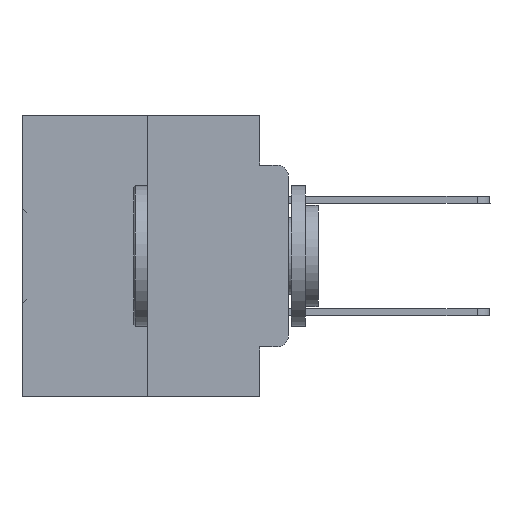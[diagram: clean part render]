
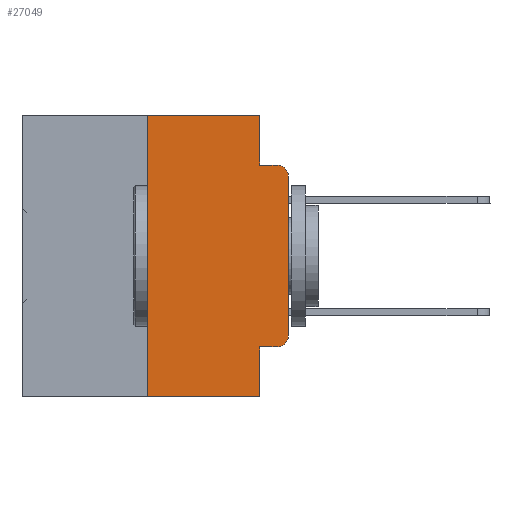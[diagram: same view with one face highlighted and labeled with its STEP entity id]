
A CAD part, left-side view. The second image highlights one B-rep face of the part: STEP entity #27049.
In plain terms, the highlighted planar face has unit normal (-1, 0, 0).
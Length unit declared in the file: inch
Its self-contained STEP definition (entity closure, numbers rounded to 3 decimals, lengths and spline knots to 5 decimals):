
#263 = CARTESIAN_POINT ( 'NONE',  ( 0., 0.051, -0.4115 ) ) ;
#491 = VERTEX_POINT ( 'NONE', #30525 ) ;
#602 = CARTESIAN_POINT ( 'NONE',  ( 0., 0.25, -0.5 ) ) ;
#1112 = DIRECTION ( 'NONE',  ( 0., 0., -1. ) ) ;
#1123 = DIRECTION ( 'NONE',  ( 0., -1., 0. ) ) ;
#1315 = ORIENTED_EDGE ( 'NONE', *, *, #19441, .T. ) ;
#2215 = CARTESIAN_POINT ( 'NONE',  ( 0., 0.02, -0.1085 ) ) ;
#2523 = DIRECTION ( 'NONE',  ( 0., 0., 1. ) ) ;
#2767 = ORIENTED_EDGE ( 'NONE', *, *, #11014, .F. ) ;
#2923 = VERTEX_POINT ( 'NONE', #30788 ) ;
#3216 = VERTEX_POINT ( 'NONE', #3576 ) ;
#3576 = CARTESIAN_POINT ( 'NONE',  ( 0., 0.02, -0.4115 ) ) ;
#4237 = EDGE_CURVE ( 'NONE', #9511, #13830, #15731, .T. ) ;
#4413 = ORIENTED_EDGE ( 'NONE', *, *, #8014, .T. ) ;
#5120 = LINE ( 'NONE', #29981, #7743 ) ;
#5161 = CARTESIAN_POINT ( 'NONE',  ( 0., 0.051, -0.4115 ) ) ;
#6084 = VERTEX_POINT ( 'NONE', #8477 ) ;
#6531 = LINE ( 'NONE', #29184, #16948 ) ;
#7331 = ORIENTED_EDGE ( 'NONE', *, *, #21489, .F. ) ;
#7436 = DIRECTION ( 'NONE',  ( 0., 0., 1. ) ) ;
#7743 = VECTOR ( 'NONE', #7436, 39.37008 ) ;
#7784 = AXIS2_PLACEMENT_3D ( 'NONE', #8228, #27696, #29920 ) ;
#8014 = EDGE_CURVE ( 'NONE', #3216, #491, #21829, .T. ) ;
#8165 = VECTOR ( 'NONE', #2523, 39.37008 ) ;
#8228 = CARTESIAN_POINT ( 'NONE',  ( 0., 0.473, 0. ) ) ;
#8248 = ORIENTED_EDGE ( 'NONE', *, *, #23022, .F. ) ;
#8477 = CARTESIAN_POINT ( 'NONE',  ( 0., 0.051, -0.0885 ) ) ;
#9511 = VERTEX_POINT ( 'NONE', #602 ) ;
#10526 = DIRECTION ( 'NONE',  ( -1., 0., 0. ) ) ;
#10883 = DIRECTION ( 'NONE',  ( 0., -1., 0. ) ) ;
#11014 = EDGE_CURVE ( 'NONE', #18075, #2923, #6531, .T. ) ;
#11150 = EDGE_CURVE ( 'NONE', #11216, #31219, #32682, .T. ) ;
#11216 = VERTEX_POINT ( 'NONE', #18666 ) ;
#11262 = EDGE_CURVE ( 'NONE', #28869, #3216, #24409, .T. ) ;
#11607 = DIRECTION ( 'NONE',  ( 0., -1., 0. ) ) ;
#11678 = LINE ( 'NONE', #14101, #14292 ) ;
#11853 = ORIENTED_EDGE ( 'NONE', *, *, #27404, .F. ) ;
#12034 = ORIENTED_EDGE ( 'NONE', *, *, #11150, .T. ) ;
#12565 = AXIS2_PLACEMENT_3D ( 'NONE', #12947, #19152, #1112 ) ;
#12947 = CARTESIAN_POINT ( 'NONE',  ( 0., 0.02, -0.3915 ) ) ;
#13374 = DIRECTION ( 'NONE',  ( 0., 0., -1. ) ) ;
#13830 = VERTEX_POINT ( 'NONE', #25325 ) ;
#14101 = CARTESIAN_POINT ( 'NONE',  ( 0., 0.051, 0. ) ) ;
#14292 = VECTOR ( 'NONE', #19574, 39.37008 ) ;
#15259 = VECTOR ( 'NONE', #10883, 39.37008 ) ;
#15731 = LINE ( 'NONE', #34508, #18341 ) ;
#16223 = PLANE ( 'NONE',  #7784 ) ;
#16948 = VECTOR ( 'NONE', #29052, 39.37008 ) ;
#18075 = VERTEX_POINT ( 'NONE', #31237 ) ;
#18341 = VECTOR ( 'NONE', #1123, 39.37008 ) ;
#18666 = CARTESIAN_POINT ( 'NONE',  ( 0., 0., -0.1085 ) ) ;
#18863 = ORIENTED_EDGE ( 'NONE', *, *, #19677, .F. ) ;
#19147 = DIRECTION ( 'NONE',  ( 0., 0., -1. ) ) ;
#19152 = DIRECTION ( 'NONE',  ( -1., 0., 0. ) ) ;
#19441 = EDGE_CURVE ( 'NONE', #491, #11216, #5120, .T. ) ;
#19447 = CARTESIAN_POINT ( 'NONE',  ( 0., 0.25, 0. ) ) ;
#19574 = DIRECTION ( 'NONE',  ( 0., 0., -1. ) ) ;
#19677 = EDGE_CURVE ( 'NONE', #9511, #18075, #32994, .T. ) ;
#21489 = EDGE_CURVE ( 'NONE', #28869, #13830, #11678, .T. ) ;
#21829 = CIRCLE ( 'NONE', #12565, 0.02 ) ;
#22908 = CARTESIAN_POINT ( 'NONE',  ( 0., 0.051, -0.0885 ) ) ;
#23022 = EDGE_CURVE ( 'NONE', #2923, #6084, #31638, .T. ) ;
#23381 = AXIS2_PLACEMENT_3D ( 'NONE', #2215, #10526, #19147 ) ;
#23522 = EDGE_LOOP ( 'NONE', ( #1315, #12034, #11853, #8248, #2767, #18863, #31347, #7331, #28934, #4413 ) ) ;
#24409 = LINE ( 'NONE', #5161, #15259 ) ;
#25325 = CARTESIAN_POINT ( 'NONE',  ( 0., 0.051, -0.5 ) ) ;
#27049 = ADVANCED_FACE ( 'NONE', ( #33118 ), #16223, .F. ) ;
#27404 = EDGE_CURVE ( 'NONE', #6084, #31219, #31792, .T. ) ;
#27427 = VECTOR ( 'NONE', #11607, 39.37008 ) ;
#27696 = DIRECTION ( 'NONE',  ( 1., 0., 0. ) ) ;
#28869 = VERTEX_POINT ( 'NONE', #263 ) ;
#28934 = ORIENTED_EDGE ( 'NONE', *, *, #11262, .T. ) ;
#29052 = DIRECTION ( 'NONE',  ( 0., -1., 0. ) ) ;
#29184 = CARTESIAN_POINT ( 'NONE',  ( 0., 0.473, 0. ) ) ;
#29920 = DIRECTION ( 'NONE',  ( 0., 0., -1. ) ) ;
#29981 = CARTESIAN_POINT ( 'NONE',  ( 0., 0., 0. ) ) ;
#30525 = CARTESIAN_POINT ( 'NONE',  ( 0., 0., -0.3915 ) ) ;
#30788 = CARTESIAN_POINT ( 'NONE',  ( 0., 0.051, 0. ) ) ;
#31219 = VERTEX_POINT ( 'NONE', #34226 ) ;
#31237 = CARTESIAN_POINT ( 'NONE',  ( 0., 0.25, 0. ) ) ;
#31347 = ORIENTED_EDGE ( 'NONE', *, *, #4237, .T. ) ;
#31638 = LINE ( 'NONE', #33112, #35553 ) ;
#31792 = LINE ( 'NONE', #22908, #27427 ) ;
#32682 = CIRCLE ( 'NONE', #23381, 0.02 ) ;
#32994 = LINE ( 'NONE', #19447, #8165 ) ;
#33112 = CARTESIAN_POINT ( 'NONE',  ( 0., 0.051, 0. ) ) ;
#33118 = FACE_OUTER_BOUND ( 'NONE', #23522, .T. ) ;
#34226 = CARTESIAN_POINT ( 'NONE',  ( 0., 0.02, -0.0885 ) ) ;
#34508 = CARTESIAN_POINT ( 'NONE',  ( 0., 0.473, -0.5 ) ) ;
#35553 = VECTOR ( 'NONE', #13374, 39.37008 ) ;
